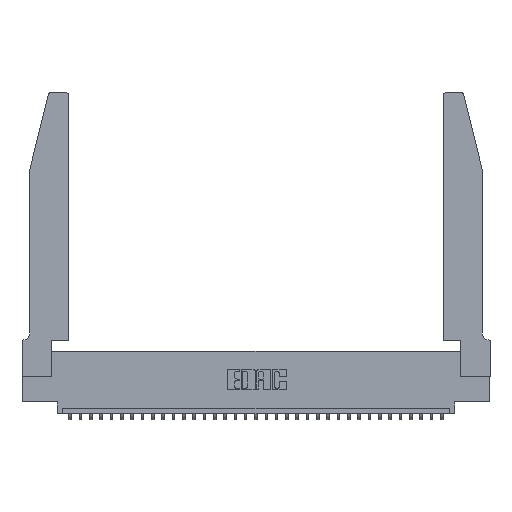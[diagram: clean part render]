
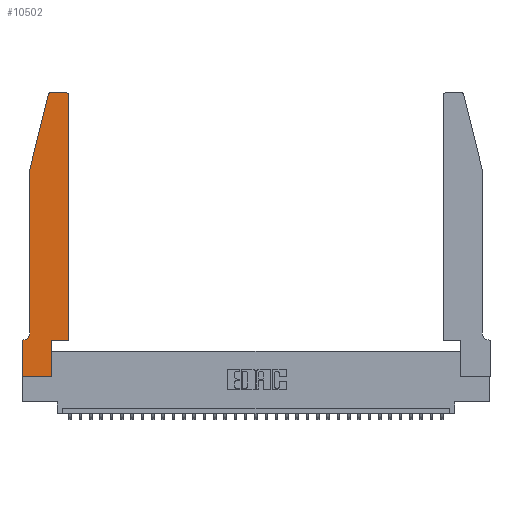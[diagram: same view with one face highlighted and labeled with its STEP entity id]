
A CAD part, top view. The second image highlights one B-rep face of the part: STEP entity #10502.
In plain terms, the highlighted planar face has unit normal (0, 0, 1).
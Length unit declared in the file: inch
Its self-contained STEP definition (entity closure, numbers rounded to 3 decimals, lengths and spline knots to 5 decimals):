
#52 = CARTESIAN_POINT ( 'NONE',  ( 0.4505, 0.35, 0.37 ) ) ;
#316 = CARTESIAN_POINT ( 'NONE',  ( 0., 0., 0.37 ) ) ;
#382 = LINE ( 'NONE', #26519, #6131 ) ;
#521 = VERTEX_POINT ( 'NONE', #20925 ) ;
#862 = AXIS2_PLACEMENT_3D ( 'NONE', #27822, #21010, #11689 ) ;
#1109 = DIRECTION ( 'NONE',  ( 0., 1., 0. ) ) ;
#1489 = CIRCLE ( 'NONE', #862, 0.03 ) ;
#2511 = DIRECTION ( 'NONE',  ( 1., 0., 0. ) ) ;
#2706 = ORIENTED_EDGE ( 'NONE', *, *, #20660, .T. ) ;
#2737 = DIRECTION ( 'NONE',  ( -1., 0., 0. ) ) ;
#2770 = DIRECTION ( 'NONE',  ( 0., -1., 0. ) ) ;
#2879 = EDGE_CURVE ( 'NONE', #3716, #28825, #13477, .T. ) ;
#2977 = EDGE_CURVE ( 'NONE', #31472, #3716, #26530, .T. ) ;
#3079 = CARTESIAN_POINT ( 'NONE',  ( 0.2605, 2.75, 0.37 ) ) ;
#3379 = CARTESIAN_POINT ( 'NONE',  ( 0., 0.35, 0.37 ) ) ;
#3716 = VERTEX_POINT ( 'NONE', #16262 ) ;
#3776 = CARTESIAN_POINT ( 'NONE',  ( 0.0055, 0.35, 0.37 ) ) ;
#3977 = EDGE_CURVE ( 'NONE', #28825, #7980, #32068, .T. ) ;
#4145 = VECTOR ( 'NONE', #2770, 39.37008 ) ;
#4158 = DIRECTION ( 'NONE',  ( 0., 1., 0. ) ) ;
#4263 = EDGE_CURVE ( 'NONE', #30180, #21535, #11410, .T. ) ;
#5097 = EDGE_CURVE ( 'NONE', #21447, #21522, #382, .T. ) ;
#5233 = CARTESIAN_POINT ( 'NONE',  ( 0.0755, 0.42, 0.37 ) ) ;
#5272 = CARTESIAN_POINT ( 'NONE',  ( 0.0755, 2., 0.37 ) ) ;
#5378 = DIRECTION ( 'NONE',  ( 0., 0., -1. ) ) ;
#6131 = VECTOR ( 'NONE', #9673, 39.37008 ) ;
#6382 = DIRECTION ( 'NONE',  ( -0.239, -0.971, 0. ) ) ;
#6633 = VECTOR ( 'NONE', #1109, 39.37008 ) ;
#6682 = CARTESIAN_POINT ( 'NONE',  ( 0.2865, 0.35, 0.37 ) ) ;
#7031 = VECTOR ( 'NONE', #31465, 39.37008 ) ;
#7743 = CARTESIAN_POINT ( 'NONE',  ( 0.25487, 2.72718, 0.37 ) ) ;
#7980 = VERTEX_POINT ( 'NONE', #17286 ) ;
#8154 = LINE ( 'NONE', #316, #10595 ) ;
#8876 = LINE ( 'NONE', #3079, #14197 ) ;
#9369 = CARTESIAN_POINT ( 'NONE',  ( 0.0055, 0.42, 0.37 ) ) ;
#9673 = DIRECTION ( 'NONE',  ( 0., -1., 0. ) ) ;
#10502 = ADVANCED_FACE ( 'NONE', ( #26125 ), #18758, .T. ) ;
#10595 = VECTOR ( 'NONE', #2511, 39.37008 ) ;
#10797 = CARTESIAN_POINT ( 'NONE',  ( 0., 0., 0.37 ) ) ;
#10861 = EDGE_CURVE ( 'NONE', #21522, #30180, #30192, .T. ) ;
#10918 = VERTEX_POINT ( 'NONE', #23257 ) ;
#11093 = CIRCLE ( 'NONE', #33014, 0.03 ) ;
#11189 = CARTESIAN_POINT ( 'NONE',  ( 0.4505, 0.35, 0.37 ) ) ;
#11410 = LINE ( 'NONE', #16313, #23210 ) ;
#11689 = DIRECTION ( 'NONE',  ( 1., 0., 0. ) ) ;
#11690 = VERTEX_POINT ( 'NONE', #7743 ) ;
#12070 = AXIS2_PLACEMENT_3D ( 'NONE', #9369, #5378, #2737 ) ;
#13477 = LINE ( 'NONE', #52, #7031 ) ;
#13782 = ORIENTED_EDGE ( 'NONE', *, *, #2977, .T. ) ;
#13871 = DIRECTION ( 'NONE',  ( -1., 0., 0. ) ) ;
#13877 = LINE ( 'NONE', #10797, #4145 ) ;
#14105 = EDGE_CURVE ( 'NONE', #18182, #10918, #8876, .T. ) ;
#14197 = VECTOR ( 'NONE', #13871, 39.37008 ) ;
#14565 = ORIENTED_EDGE ( 'NONE', *, *, #14105, .T. ) ;
#14942 = ORIENTED_EDGE ( 'NONE', *, *, #2879, .T. ) ;
#15406 = CARTESIAN_POINT ( 'NONE',  ( 0., 0.35, 0.37 ) ) ;
#16080 = CARTESIAN_POINT ( 'NONE',  ( 0.0755, 2., 0.37 ) ) ;
#16262 = CARTESIAN_POINT ( 'NONE',  ( 0.2865, 0.35, 0.37 ) ) ;
#16313 = CARTESIAN_POINT ( 'NONE',  ( 0.0755, 0.35, 0.37 ) ) ;
#16886 = DIRECTION ( 'NONE',  ( -1., 0., 0. ) ) ;
#17286 = CARTESIAN_POINT ( 'NONE',  ( 0.4505, 2.72, 0.37 ) ) ;
#17421 = DIRECTION ( 'NONE',  ( 0., 0., 1. ) ) ;
#17474 = ORIENTED_EDGE ( 'NONE', *, *, #4263, .T. ) ;
#17724 = ORIENTED_EDGE ( 'NONE', *, *, #3977, .T. ) ;
#18040 = VECTOR ( 'NONE', #4158, 39.37008 ) ;
#18182 = VERTEX_POINT ( 'NONE', #22121 ) ;
#18215 = CARTESIAN_POINT ( 'NONE',  ( 0.4505, 0.35, 0.37 ) ) ;
#18758 = PLANE ( 'NONE',  #25940 ) ;
#18870 = DIRECTION ( 'NONE',  ( 1., 0., 0. ) ) ;
#19732 = VECTOR ( 'NONE', #6382, 39.37008 ) ;
#20023 = CARTESIAN_POINT ( 'NONE',  ( 0.284, 2.72, 0.37 ) ) ;
#20446 = ORIENTED_EDGE ( 'NONE', *, *, #26972, .T. ) ;
#20660 = EDGE_CURVE ( 'NONE', #521, #31472, #8154, .T. ) ;
#20925 = CARTESIAN_POINT ( 'NONE',  ( 0., 0., 0.37 ) ) ;
#21010 = DIRECTION ( 'NONE',  ( 0., 0., 1. ) ) ;
#21447 = VERTEX_POINT ( 'NONE', #5272 ) ;
#21522 = VERTEX_POINT ( 'NONE', #5233 ) ;
#21535 = VERTEX_POINT ( 'NONE', #15406 ) ;
#21605 = ORIENTED_EDGE ( 'NONE', *, *, #26860, .T. ) ;
#22121 = CARTESIAN_POINT ( 'NONE',  ( 0.4205, 2.75, 0.37 ) ) ;
#22830 = ORIENTED_EDGE ( 'NONE', *, *, #32149, .T. ) ;
#23210 = VECTOR ( 'NONE', #16886, 39.37008 ) ;
#23257 = CARTESIAN_POINT ( 'NONE',  ( 0.284, 2.75, 0.37 ) ) ;
#24698 = EDGE_LOOP ( 'NONE', ( #14565, #33425, #21605, #31162, #31376, #17474, #22830, #2706, #13782, #14942, #17724, #20446 ) ) ;
#25940 = AXIS2_PLACEMENT_3D ( 'NONE', #3379, #31745, #18870 ) ;
#26125 = FACE_OUTER_BOUND ( 'NONE', #24698, .T. ) ;
#26519 = CARTESIAN_POINT ( 'NONE',  ( 0.0755, 2., 0.37 ) ) ;
#26530 = LINE ( 'NONE', #6682, #18040 ) ;
#26860 = EDGE_CURVE ( 'NONE', #11690, #21447, #29437, .T. ) ;
#26972 = EDGE_CURVE ( 'NONE', #7980, #18182, #1489, .T. ) ;
#27822 = CARTESIAN_POINT ( 'NONE',  ( 0.4205, 2.72, 0.37 ) ) ;
#28069 = CARTESIAN_POINT ( 'NONE',  ( 0.2865, 0., 0.37 ) ) ;
#28825 = VERTEX_POINT ( 'NONE', #18215 ) ;
#29298 = DIRECTION ( 'NONE',  ( 1., 0., 0. ) ) ;
#29437 = LINE ( 'NONE', #16080, #19732 ) ;
#30180 = VERTEX_POINT ( 'NONE', #3776 ) ;
#30192 = CIRCLE ( 'NONE', #12070, 0.07 ) ;
#31039 = EDGE_CURVE ( 'NONE', #10918, #11690, #11093, .T. ) ;
#31162 = ORIENTED_EDGE ( 'NONE', *, *, #5097, .T. ) ;
#31376 = ORIENTED_EDGE ( 'NONE', *, *, #10861, .T. ) ;
#31465 = DIRECTION ( 'NONE',  ( 1., 0., 0. ) ) ;
#31472 = VERTEX_POINT ( 'NONE', #28069 ) ;
#31745 = DIRECTION ( 'NONE',  ( 0., 0., 1. ) ) ;
#32068 = LINE ( 'NONE', #11189, #6633 ) ;
#32149 = EDGE_CURVE ( 'NONE', #21535, #521, #13877, .T. ) ;
#33014 = AXIS2_PLACEMENT_3D ( 'NONE', #20023, #17421, #29298 ) ;
#33425 = ORIENTED_EDGE ( 'NONE', *, *, #31039, .T. ) ;
